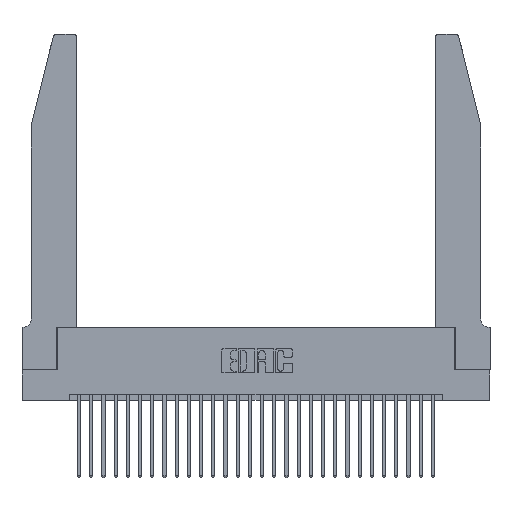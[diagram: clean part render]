
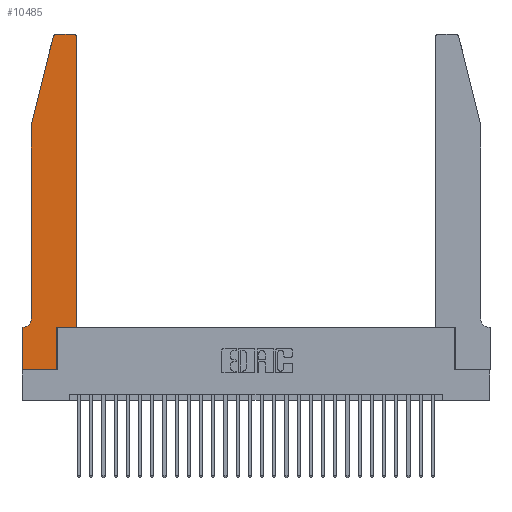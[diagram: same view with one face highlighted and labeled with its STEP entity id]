
A CAD part, top view. The second image highlights one B-rep face of the part: STEP entity #10485.
In plain terms, the highlighted planar face has unit normal (0, 0, 1).
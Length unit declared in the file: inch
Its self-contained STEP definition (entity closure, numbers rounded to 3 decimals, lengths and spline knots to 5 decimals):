
#309 = ORIENTED_EDGE ( 'NONE', *, *, #28001, .T. ) ;
#455 = ORIENTED_EDGE ( 'NONE', *, *, #2956, .T. ) ;
#673 = EDGE_CURVE ( 'NONE', #3565, #16183, #16449, .T. ) ;
#684 = VERTEX_POINT ( 'NONE', #26117 ) ;
#910 = CIRCLE ( 'NONE', #24447, 0.03 ) ;
#1687 = CARTESIAN_POINT ( 'NONE',  ( 0.284, 2.75, 0.37 ) ) ;
#2485 = DIRECTION ( 'NONE',  ( -1., 0., 0. ) ) ;
#2486 = VECTOR ( 'NONE', #11188, 39.37008 ) ;
#2816 = PLANE ( 'NONE',  #4573 ) ;
#2835 = CARTESIAN_POINT ( 'NONE',  ( 0.0755, 2., 0.37 ) ) ;
#2956 = EDGE_CURVE ( 'NONE', #23900, #10947, #16376, .T. ) ;
#3565 = VERTEX_POINT ( 'NONE', #17550 ) ;
#3671 = EDGE_CURVE ( 'NONE', #4142, #23150, #10522, .T. ) ;
#3761 = ORIENTED_EDGE ( 'NONE', *, *, #12491, .T. ) ;
#4142 = VERTEX_POINT ( 'NONE', #18300 ) ;
#4523 = CARTESIAN_POINT ( 'NONE',  ( 0.284, 2.72, 0.37 ) ) ;
#4573 = AXIS2_PLACEMENT_3D ( 'NONE', #26270, #12434, #16158 ) ;
#4705 = AXIS2_PLACEMENT_3D ( 'NONE', #4523, #29907, #11713 ) ;
#5529 = ORIENTED_EDGE ( 'NONE', *, *, #8041, .T. ) ;
#6067 = ORIENTED_EDGE ( 'NONE', *, *, #29026, .T. ) ;
#6409 = VECTOR ( 'NONE', #27065, 39.37008 ) ;
#6411 = ORIENTED_EDGE ( 'NONE', *, *, #24184, .T. ) ;
#6913 = ORIENTED_EDGE ( 'NONE', *, *, #673, .T. ) ;
#8041 = EDGE_CURVE ( 'NONE', #19026, #3565, #16833, .T. ) ;
#8101 = VERTEX_POINT ( 'NONE', #16502 ) ;
#8178 = CARTESIAN_POINT ( 'NONE',  ( 0., 0., 0.37 ) ) ;
#8396 = DIRECTION ( 'NONE',  ( 0., 1., 0. ) ) ;
#9013 = DIRECTION ( 'NONE',  ( 0., 0., 1. ) ) ;
#9031 = CARTESIAN_POINT ( 'NONE',  ( 0.2605, 2.75, 0.37 ) ) ;
#9525 = CARTESIAN_POINT ( 'NONE',  ( 0.0755, 0.35, 0.37 ) ) ;
#9571 = LINE ( 'NONE', #26534, #26945 ) ;
#10485 = ADVANCED_FACE ( 'NONE', ( #19562 ), #2816, .T. ) ;
#10522 = LINE ( 'NONE', #14923, #21430 ) ;
#10610 = DIRECTION ( 'NONE',  ( 1., 0., 0. ) ) ;
#10947 = VERTEX_POINT ( 'NONE', #26543 ) ;
#11188 = DIRECTION ( 'NONE',  ( 0., -1., 0. ) ) ;
#11346 = CARTESIAN_POINT ( 'NONE',  ( 0.4505, 0.35, 0.37 ) ) ;
#11659 = DIRECTION ( 'NONE',  ( 0., 0., -1. ) ) ;
#11713 = DIRECTION ( 'NONE',  ( 1., 0., 0. ) ) ;
#11876 = DIRECTION ( 'NONE',  ( 0., -1., 0. ) ) ;
#11879 = DIRECTION ( 'NONE',  ( -1., 0., 0. ) ) ;
#12434 = DIRECTION ( 'NONE',  ( 0., 0., 1. ) ) ;
#12491 = EDGE_CURVE ( 'NONE', #24776, #14752, #12926, .T. ) ;
#12926 = CIRCLE ( 'NONE', #4705, 0.03 ) ;
#13645 = EDGE_CURVE ( 'NONE', #684, #19026, #22293, .T. ) ;
#13707 = DIRECTION ( 'NONE',  ( 1., 0., 0. ) ) ;
#14020 = EDGE_CURVE ( 'NONE', #23150, #18070, #9571, .T. ) ;
#14505 = CARTESIAN_POINT ( 'NONE',  ( 0.0755, 2., 0.37 ) ) ;
#14622 = ORIENTED_EDGE ( 'NONE', *, *, #14020, .T. ) ;
#14715 = VECTOR ( 'NONE', #26089, 39.37008 ) ;
#14752 = VERTEX_POINT ( 'NONE', #24530 ) ;
#14881 = VECTOR ( 'NONE', #18366, 39.37008 ) ;
#14923 = CARTESIAN_POINT ( 'NONE',  ( 0.4505, 0.35, 0.37 ) ) ;
#15245 = CARTESIAN_POINT ( 'NONE',  ( 0., 0., 0.37 ) ) ;
#16107 = VECTOR ( 'NONE', #11876, 39.37008 ) ;
#16158 = DIRECTION ( 'NONE',  ( 1., 0., 0. ) ) ;
#16183 = VERTEX_POINT ( 'NONE', #16535 ) ;
#16356 = EDGE_CURVE ( 'NONE', #10947, #4142, #24935, .T. ) ;
#16376 = LINE ( 'NONE', #8178, #28702 ) ;
#16449 = LINE ( 'NONE', #9525, #25853 ) ;
#16502 = CARTESIAN_POINT ( 'NONE',  ( 0.4205, 2.75, 0.37 ) ) ;
#16535 = CARTESIAN_POINT ( 'NONE',  ( 0., 0.35, 0.37 ) ) ;
#16833 = CIRCLE ( 'NONE', #28797, 0.07 ) ;
#16878 = CARTESIAN_POINT ( 'NONE',  ( 0., 0., 0.37 ) ) ;
#17069 = CARTESIAN_POINT ( 'NONE',  ( 0.4505, 2.72, 0.37 ) ) ;
#17550 = CARTESIAN_POINT ( 'NONE',  ( 0.0055, 0.35, 0.37 ) ) ;
#17906 = ORIENTED_EDGE ( 'NONE', *, *, #25372, .T. ) ;
#18070 = VERTEX_POINT ( 'NONE', #17069 ) ;
#18300 = CARTESIAN_POINT ( 'NONE',  ( 0.2865, 0.35, 0.37 ) ) ;
#18366 = DIRECTION ( 'NONE',  ( -1., 0., 0. ) ) ;
#18652 = CARTESIAN_POINT ( 'NONE',  ( 0.0055, 0.42, 0.37 ) ) ;
#19026 = VERTEX_POINT ( 'NONE', #21442 ) ;
#19562 = FACE_OUTER_BOUND ( 'NONE', #28422, .T. ) ;
#20026 = ORIENTED_EDGE ( 'NONE', *, *, #13645, .T. ) ;
#21430 = VECTOR ( 'NONE', #24460, 39.37008 ) ;
#21442 = CARTESIAN_POINT ( 'NONE',  ( 0.0755, 0.42, 0.37 ) ) ;
#22293 = LINE ( 'NONE', #14505, #16107 ) ;
#22729 = LINE ( 'NONE', #2835, #14715 ) ;
#23150 = VERTEX_POINT ( 'NONE', #11346 ) ;
#23900 = VERTEX_POINT ( 'NONE', #16878 ) ;
#24184 = EDGE_CURVE ( 'NONE', #16183, #23900, #26342, .T. ) ;
#24447 = AXIS2_PLACEMENT_3D ( 'NONE', #29753, #9013, #13707 ) ;
#24460 = DIRECTION ( 'NONE',  ( 1., 0., 0. ) ) ;
#24530 = CARTESIAN_POINT ( 'NONE',  ( 0.25487, 2.72718, 0.37 ) ) ;
#24776 = VERTEX_POINT ( 'NONE', #1687 ) ;
#24935 = LINE ( 'NONE', #27754, #6409 ) ;
#24978 = ORIENTED_EDGE ( 'NONE', *, *, #16356, .T. ) ;
#25372 = EDGE_CURVE ( 'NONE', #8101, #24776, #27208, .T. ) ;
#25853 = VECTOR ( 'NONE', #11879, 39.37008 ) ;
#26089 = DIRECTION ( 'NONE',  ( -0.239, -0.971, 0. ) ) ;
#26117 = CARTESIAN_POINT ( 'NONE',  ( 0.0755, 2., 0.37 ) ) ;
#26270 = CARTESIAN_POINT ( 'NONE',  ( 0., 0.35, 0.37 ) ) ;
#26342 = LINE ( 'NONE', #15245, #2486 ) ;
#26534 = CARTESIAN_POINT ( 'NONE',  ( 0.4505, 0.35, 0.37 ) ) ;
#26543 = CARTESIAN_POINT ( 'NONE',  ( 0.2865, 0., 0.37 ) ) ;
#26945 = VECTOR ( 'NONE', #8396, 39.37008 ) ;
#27065 = DIRECTION ( 'NONE',  ( 0., 1., 0. ) ) ;
#27208 = LINE ( 'NONE', #9031, #14881 ) ;
#27754 = CARTESIAN_POINT ( 'NONE',  ( 0.2865, 0.35, 0.37 ) ) ;
#28001 = EDGE_CURVE ( 'NONE', #14752, #684, #22729, .T. ) ;
#28422 = EDGE_LOOP ( 'NONE', ( #17906, #3761, #309, #20026, #5529, #6913, #6411, #455, #24978, #28753, #14622, #6067 ) ) ;
#28702 = VECTOR ( 'NONE', #10610, 39.37008 ) ;
#28753 = ORIENTED_EDGE ( 'NONE', *, *, #3671, .T. ) ;
#28797 = AXIS2_PLACEMENT_3D ( 'NONE', #18652, #11659, #2485 ) ;
#29026 = EDGE_CURVE ( 'NONE', #18070, #8101, #910, .T. ) ;
#29753 = CARTESIAN_POINT ( 'NONE',  ( 0.4205, 2.72, 0.37 ) ) ;
#29907 = DIRECTION ( 'NONE',  ( 0., 0., 1. ) ) ;
